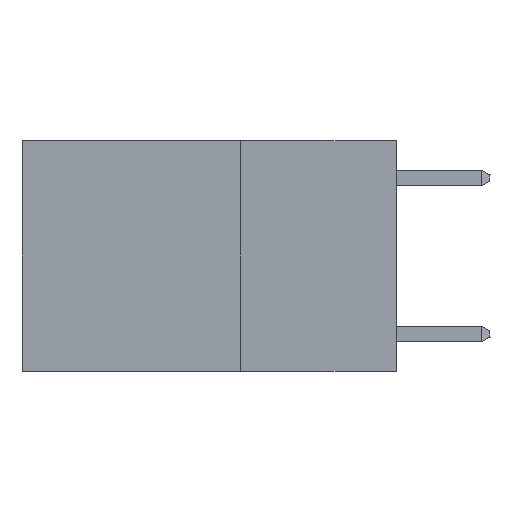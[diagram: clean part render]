
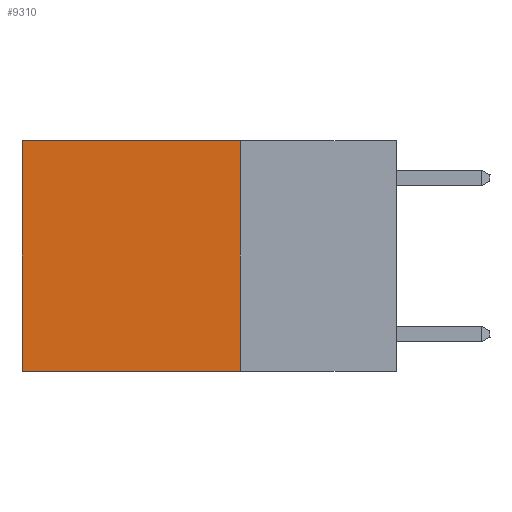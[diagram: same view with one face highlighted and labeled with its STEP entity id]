
A CAD part, left-side view. The second image highlights one B-rep face of the part: STEP entity #9310.
In plain terms, the highlighted planar face has unit normal (-1, 0, 0).
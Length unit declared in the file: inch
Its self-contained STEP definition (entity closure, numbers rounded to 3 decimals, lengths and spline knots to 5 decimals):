
#315 = CARTESIAN_POINT ( 'NONE',  ( 0.2625, 0.25, -0.37 ) ) ;
#355 = VERTEX_POINT ( 'NONE', #315 ) ;
#1609 = CARTESIAN_POINT ( 'NONE',  ( 0.2625, 0.25, 0. ) ) ;
#1713 = EDGE_CURVE ( 'NONE', #4038, #3228, #7734, .T. ) ;
#2816 = EDGE_CURVE ( 'NONE', #355, #11800, #8180, .T. ) ;
#3054 = EDGE_CURVE ( 'NONE', #4038, #355, #9862, .T. ) ;
#3228 = VERTEX_POINT ( 'NONE', #12390 ) ;
#3584 = AXIS2_PLACEMENT_3D ( 'NONE', #6938, #11114, #8969 ) ;
#4038 = VERTEX_POINT ( 'NONE', #1609 ) ;
#4567 = DIRECTION ( 'NONE',  ( 0., 0., -1. ) ) ;
#5419 = VECTOR ( 'NONE', #5657, 39.37008 ) ;
#5657 = DIRECTION ( 'NONE',  ( 0., 1., 0. ) ) ;
#5724 = EDGE_CURVE ( 'NONE', #3228, #11800, #8055, .T. ) ;
#5820 = EDGE_LOOP ( 'NONE', ( #6214, #8634, #7232, #13340 ) ) ;
#5907 = DIRECTION ( 'NONE',  ( 0., 0., -1. ) ) ;
#6024 = VECTOR ( 'NONE', #4567, 39.37008 ) ;
#6214 = ORIENTED_EDGE ( 'NONE', *, *, #5724, .T. ) ;
#6477 = CARTESIAN_POINT ( 'NONE',  ( 0.2625, 0.6, -0.37 ) ) ;
#6725 = CARTESIAN_POINT ( 'NONE',  ( 0.2625, 0.25, 0. ) ) ;
#6938 = CARTESIAN_POINT ( 'NONE',  ( 0.2625, 0.25, 0. ) ) ;
#7232 = ORIENTED_EDGE ( 'NONE', *, *, #3054, .F. ) ;
#7734 = LINE ( 'NONE', #12009, #5419 ) ;
#8055 = LINE ( 'NONE', #12348, #13005 ) ;
#8180 = LINE ( 'NONE', #9302, #10664 ) ;
#8634 = ORIENTED_EDGE ( 'NONE', *, *, #2816, .F. ) ;
#8896 = PLANE ( 'NONE',  #3584 ) ;
#8969 = DIRECTION ( 'NONE',  ( 0., 0., -1. ) ) ;
#9302 = CARTESIAN_POINT ( 'NONE',  ( 0.2625, 0.25, -0.37 ) ) ;
#9310 = ADVANCED_FACE ( 'NONE', ( #10089 ), #8896, .F. ) ;
#9862 = LINE ( 'NONE', #6725, #6024 ) ;
#10089 = FACE_OUTER_BOUND ( 'NONE', #5820, .T. ) ;
#10664 = VECTOR ( 'NONE', #13603, 39.37008 ) ;
#11114 = DIRECTION ( 'NONE',  ( 1., 0., 0. ) ) ;
#11800 = VERTEX_POINT ( 'NONE', #6477 ) ;
#12009 = CARTESIAN_POINT ( 'NONE',  ( 0.2625, 0.25, 0. ) ) ;
#12348 = CARTESIAN_POINT ( 'NONE',  ( 0.2625, 0.6, 0. ) ) ;
#12390 = CARTESIAN_POINT ( 'NONE',  ( 0.2625, 0.6, 0. ) ) ;
#13005 = VECTOR ( 'NONE', #5907, 39.37008 ) ;
#13340 = ORIENTED_EDGE ( 'NONE', *, *, #1713, .T. ) ;
#13603 = DIRECTION ( 'NONE',  ( 0., 1., 0. ) ) ;
